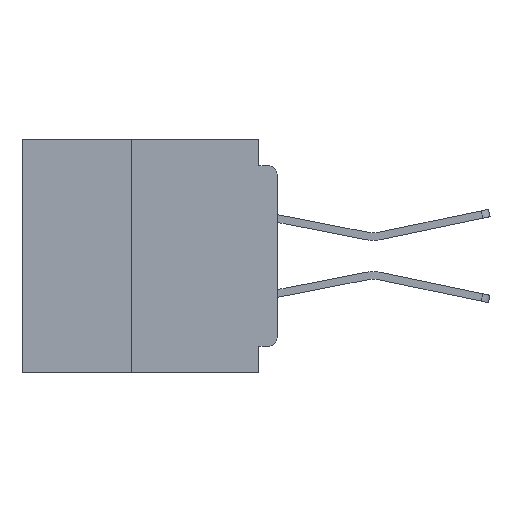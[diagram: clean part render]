
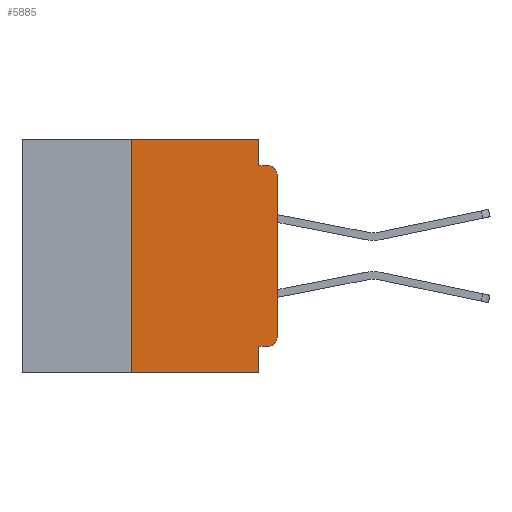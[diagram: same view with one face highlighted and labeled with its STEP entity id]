
A CAD part, left-side view. The second image highlights one B-rep face of the part: STEP entity #5885.
In plain terms, the highlighted planar face has unit normal (-1, 0, 0).
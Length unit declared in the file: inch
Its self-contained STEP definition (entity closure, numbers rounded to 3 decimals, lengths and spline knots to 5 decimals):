
#2158 = CARTESIAN_POINT ( 'NONE',  ( 0., 0.031, 0. ) ) ;
#2552 = CARTESIAN_POINT ( 'NONE',  ( 0., 0.031, -0.355 ) ) ;
#3081 = LINE ( 'NONE', #6892, #22657 ) ;
#3408 = LINE ( 'NONE', #19525, #33267 ) ;
#3671 = VECTOR ( 'NONE', #35798, 39.37008 ) ;
#4069 = LINE ( 'NONE', #12187, #32701 ) ;
#4366 = VERTEX_POINT ( 'NONE', #14692 ) ;
#4512 = DIRECTION ( 'NONE',  ( 0., 0., 1. ) ) ;
#4933 = VECTOR ( 'NONE', #13161, 39.37008 ) ;
#5885 = ADVANCED_FACE ( 'NONE', ( #21115 ), #47377, .F. ) ;
#6139 = EDGE_LOOP ( 'NONE', ( #11681, #47945, #12535, #32060, #32233, #26378, #15469, #26214, #21196, #25736 ) ) ;
#6892 = CARTESIAN_POINT ( 'NONE',  ( 0., 0.031, -0.4 ) ) ;
#7492 = CARTESIAN_POINT ( 'NONE',  ( 0., 0.015, -0.34 ) ) ;
#8476 = VERTEX_POINT ( 'NONE', #2158 ) ;
#9365 = EDGE_CURVE ( 'NONE', #27153, #9800, #34208, .T. ) ;
#9373 = EDGE_CURVE ( 'NONE', #25581, #40079, #44426, .T. ) ;
#9800 = VERTEX_POINT ( 'NONE', #2552 ) ;
#9867 = CARTESIAN_POINT ( 'NONE',  ( 0., 0.25, 0. ) ) ;
#10438 = CARTESIAN_POINT ( 'NONE',  ( 0., 0., -0.06 ) ) ;
#10726 = LINE ( 'NONE', #45942, #29060 ) ;
#10815 = DIRECTION ( 'NONE',  ( 0., 0., -1. ) ) ;
#11168 = DIRECTION ( 'NONE',  ( 0., 0., 1. ) ) ;
#11411 = DIRECTION ( 'NONE',  ( 0., 0., -1. ) ) ;
#11482 = DIRECTION ( 'NONE',  ( 0., 1., 0. ) ) ;
#11656 = CARTESIAN_POINT ( 'NONE',  ( 0., 0.015, -0.06 ) ) ;
#11681 = ORIENTED_EDGE ( 'NONE', *, *, #19124, .T. ) ;
#12187 = CARTESIAN_POINT ( 'NONE',  ( 0., 0.25, -0.4 ) ) ;
#12265 = VECTOR ( 'NONE', #11482, 39.37008 ) ;
#12535 = ORIENTED_EDGE ( 'NONE', *, *, #46471, .F. ) ;
#12650 = DIRECTION ( 'NONE',  ( 0., 0., -1. ) ) ;
#13011 = VERTEX_POINT ( 'NONE', #23029 ) ;
#13161 = DIRECTION ( 'NONE',  ( 0., -1., 0. ) ) ;
#13264 = LINE ( 'NONE', #41591, #32776 ) ;
#14692 = CARTESIAN_POINT ( 'NONE',  ( 0., 0., -0.34 ) ) ;
#15395 = CARTESIAN_POINT ( 'NONE',  ( 0., 0., -0.355 ) ) ;
#15469 = ORIENTED_EDGE ( 'NONE', *, *, #43102, .T. ) ;
#15563 = DIRECTION ( 'NONE',  ( 0., 0., -1. ) ) ;
#15579 = DIRECTION ( 'NONE',  ( 0., -1., 0. ) ) ;
#19124 = EDGE_CURVE ( 'NONE', #4366, #25581, #10726, .T. ) ;
#19525 = CARTESIAN_POINT ( 'NONE',  ( 0., 0.437, -0.4 ) ) ;
#20313 = CARTESIAN_POINT ( 'NONE',  ( 0., 0.437, 0. ) ) ;
#20931 = CIRCLE ( 'NONE', #22922, 0.015 ) ;
#21115 = FACE_OUTER_BOUND ( 'NONE', #6139, .T. ) ;
#21196 = ORIENTED_EDGE ( 'NONE', *, *, #9365, .F. ) ;
#22147 = DIRECTION ( 'NONE',  ( 0., 0., -1. ) ) ;
#22451 = EDGE_CURVE ( 'NONE', #9800, #28701, #3081, .T. ) ;
#22657 = VECTOR ( 'NONE', #10815, 39.37008 ) ;
#22922 = AXIS2_PLACEMENT_3D ( 'NONE', #7492, #34767, #11411 ) ;
#23029 = CARTESIAN_POINT ( 'NONE',  ( 0., 0.031, -0.045 ) ) ;
#24009 = AXIS2_PLACEMENT_3D ( 'NONE', #28208, #35987, #12650 ) ;
#25581 = VERTEX_POINT ( 'NONE', #10438 ) ;
#25736 = ORIENTED_EDGE ( 'NONE', *, *, #30728, .T. ) ;
#25805 = VERTEX_POINT ( 'NONE', #9867 ) ;
#25908 = VERTEX_POINT ( 'NONE', #41775 ) ;
#26214 = ORIENTED_EDGE ( 'NONE', *, *, #22451, .F. ) ;
#26378 = ORIENTED_EDGE ( 'NONE', *, *, #38203, .F. ) ;
#27153 = VERTEX_POINT ( 'NONE', #45883 ) ;
#28208 = CARTESIAN_POINT ( 'NONE',  ( 0., 0.437, 0. ) ) ;
#28701 = VERTEX_POINT ( 'NONE', #47252 ) ;
#29060 = VECTOR ( 'NONE', #11168, 39.37008 ) ;
#30728 = EDGE_CURVE ( 'NONE', #27153, #4366, #20931, .T. ) ;
#32060 = ORIENTED_EDGE ( 'NONE', *, *, #33505, .F. ) ;
#32233 = ORIENTED_EDGE ( 'NONE', *, *, #46992, .F. ) ;
#32701 = VECTOR ( 'NONE', #4512, 39.37008 ) ;
#32776 = VECTOR ( 'NONE', #22147, 39.37008 ) ;
#33267 = VECTOR ( 'NONE', #15579, 39.37008 ) ;
#33505 = EDGE_CURVE ( 'NONE', #8476, #13011, #13264, .T. ) ;
#33528 = LINE ( 'NONE', #20313, #3671 ) ;
#34208 = LINE ( 'NONE', #15395, #12265 ) ;
#34767 = DIRECTION ( 'NONE',  ( -1., 0., 0. ) ) ;
#35798 = DIRECTION ( 'NONE',  ( 0., -1., 0. ) ) ;
#35987 = DIRECTION ( 'NONE',  ( 1., 0., 0. ) ) ;
#36035 = LINE ( 'NONE', #36521, #4933 ) ;
#36521 = CARTESIAN_POINT ( 'NONE',  ( 0., 0., -0.045 ) ) ;
#38203 = EDGE_CURVE ( 'NONE', #25908, #25805, #4069, .T. ) ;
#38878 = DIRECTION ( 'NONE',  ( -1., 0., 0. ) ) ;
#40012 = AXIS2_PLACEMENT_3D ( 'NONE', #11656, #38878, #15563 ) ;
#40079 = VERTEX_POINT ( 'NONE', #43038 ) ;
#41591 = CARTESIAN_POINT ( 'NONE',  ( 0., 0.031, 0. ) ) ;
#41775 = CARTESIAN_POINT ( 'NONE',  ( 0., 0.25, -0.4 ) ) ;
#43038 = CARTESIAN_POINT ( 'NONE',  ( 0., 0.015, -0.045 ) ) ;
#43102 = EDGE_CURVE ( 'NONE', #25908, #28701, #3408, .T. ) ;
#44426 = CIRCLE ( 'NONE', #40012, 0.015 ) ;
#45883 = CARTESIAN_POINT ( 'NONE',  ( 0., 0.015, -0.355 ) ) ;
#45942 = CARTESIAN_POINT ( 'NONE',  ( 0., 0., 0. ) ) ;
#46471 = EDGE_CURVE ( 'NONE', #13011, #40079, #36035, .T. ) ;
#46992 = EDGE_CURVE ( 'NONE', #25805, #8476, #33528, .T. ) ;
#47252 = CARTESIAN_POINT ( 'NONE',  ( 0., 0.031, -0.4 ) ) ;
#47377 = PLANE ( 'NONE',  #24009 ) ;
#47945 = ORIENTED_EDGE ( 'NONE', *, *, #9373, .T. ) ;
